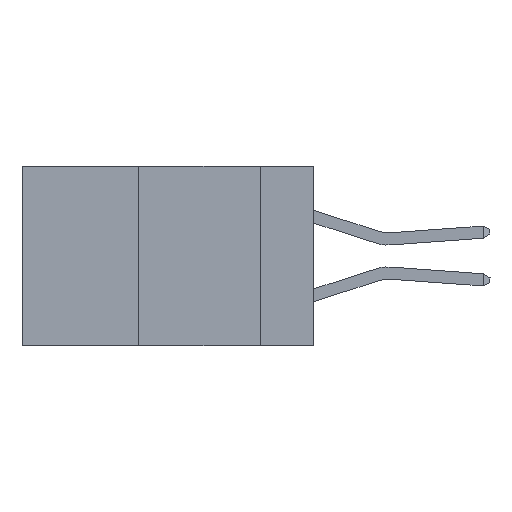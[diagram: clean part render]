
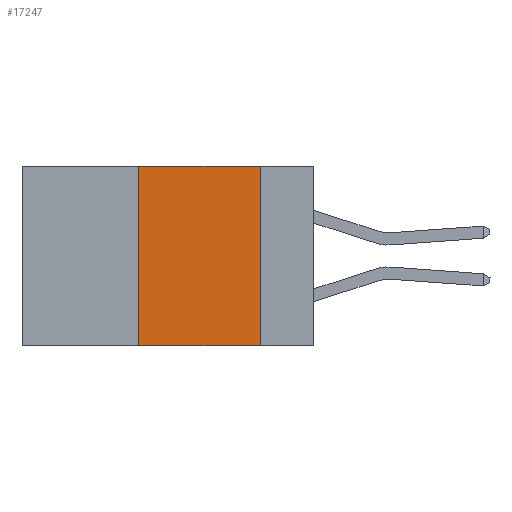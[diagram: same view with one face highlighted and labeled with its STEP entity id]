
A CAD part, left-side view. The second image highlights one B-rep face of the part: STEP entity #17247.
In plain terms, the highlighted planar face has unit normal (-1, 0, 0).
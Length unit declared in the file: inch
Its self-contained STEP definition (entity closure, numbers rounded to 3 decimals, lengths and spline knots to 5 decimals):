
#815 = LINE ( 'NONE', #1330, #13939 ) ;
#1149 = VECTOR ( 'NONE', #6874, 39.37008 ) ;
#1330 = CARTESIAN_POINT ( 'NONE',  ( 0., 0.6, -0.37 ) ) ;
#1697 = LINE ( 'NONE', #20444, #1149 ) ;
#2490 = EDGE_CURVE ( 'NONE', #10662, #2667, #21961, .T. ) ;
#2667 = VERTEX_POINT ( 'NONE', #21866 ) ;
#3050 = DIRECTION ( 'NONE',  ( 0., -1., 0. ) ) ;
#3384 = VERTEX_POINT ( 'NONE', #15147 ) ;
#3407 = EDGE_CURVE ( 'NONE', #3384, #5925, #16957, .T. ) ;
#3609 = DIRECTION ( 'NONE',  ( 1., 0., 0. ) ) ;
#3928 = VECTOR ( 'NONE', #8535, 39.37008 ) ;
#4520 = CARTESIAN_POINT ( 'NONE',  ( 0., 0.11, 0. ) ) ;
#4635 = ORIENTED_EDGE ( 'NONE', *, *, #16498, .T. ) ;
#5159 = AXIS2_PLACEMENT_3D ( 'NONE', #20512, #3609, #15552 ) ;
#5925 = VERTEX_POINT ( 'NONE', #15407 ) ;
#6874 = DIRECTION ( 'NONE',  ( 0., -1., 0. ) ) ;
#8367 = ORIENTED_EDGE ( 'NONE', *, *, #3407, .F. ) ;
#8521 = CARTESIAN_POINT ( 'NONE',  ( 0., 0.11, 0. ) ) ;
#8535 = DIRECTION ( 'NONE',  ( 0., 0., -1. ) ) ;
#8665 = PLANE ( 'NONE',  #5159 ) ;
#10144 = DIRECTION ( 'NONE',  ( 0., 0., 1. ) ) ;
#10662 = VERTEX_POINT ( 'NONE', #4520 ) ;
#10929 = EDGE_LOOP ( 'NONE', ( #15575, #16590, #8367, #4635 ) ) ;
#12480 = VECTOR ( 'NONE', #10144, 39.37008 ) ;
#13939 = VECTOR ( 'NONE', #3050, 39.37008 ) ;
#15147 = CARTESIAN_POINT ( 'NONE',  ( 0., 0.36, -0.37 ) ) ;
#15407 = CARTESIAN_POINT ( 'NONE',  ( 0., 0.36, 0. ) ) ;
#15552 = DIRECTION ( 'NONE',  ( 0., 0., -1. ) ) ;
#15575 = ORIENTED_EDGE ( 'NONE', *, *, #2490, .F. ) ;
#16498 = EDGE_CURVE ( 'NONE', #3384, #2667, #815, .T. ) ;
#16590 = ORIENTED_EDGE ( 'NONE', *, *, #21622, .F. ) ;
#16957 = LINE ( 'NONE', #18554, #12480 ) ;
#17247 = ADVANCED_FACE ( 'NONE', ( #20434 ), #8665, .F. ) ;
#18554 = CARTESIAN_POINT ( 'NONE',  ( 0., 0.36, 0. ) ) ;
#20434 = FACE_OUTER_BOUND ( 'NONE', #10929, .T. ) ;
#20444 = CARTESIAN_POINT ( 'NONE',  ( 0., 0.6, 0. ) ) ;
#20512 = CARTESIAN_POINT ( 'NONE',  ( 0., 0.6, 0. ) ) ;
#21622 = EDGE_CURVE ( 'NONE', #5925, #10662, #1697, .T. ) ;
#21866 = CARTESIAN_POINT ( 'NONE',  ( 0., 0.11, -0.37 ) ) ;
#21961 = LINE ( 'NONE', #8521, #3928 ) ;
